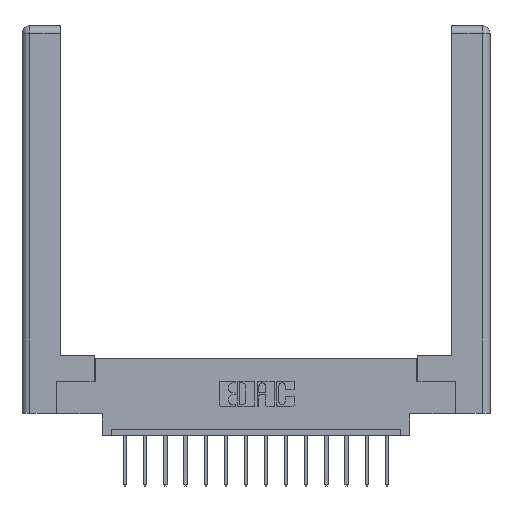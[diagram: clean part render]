
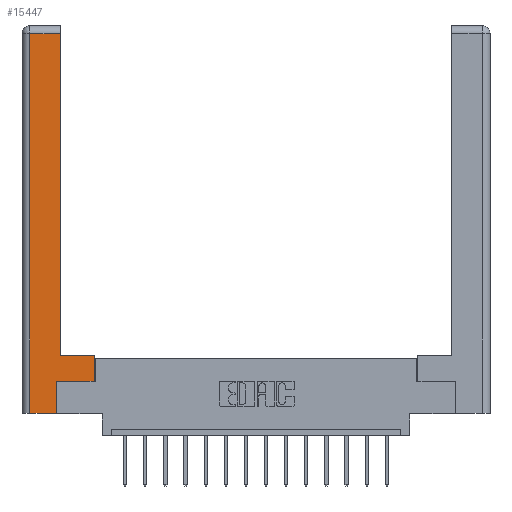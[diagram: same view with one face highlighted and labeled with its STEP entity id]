
A CAD part, top view. The second image highlights one B-rep face of the part: STEP entity #15447.
In plain terms, the highlighted planar face has unit normal (0, 0, 1).
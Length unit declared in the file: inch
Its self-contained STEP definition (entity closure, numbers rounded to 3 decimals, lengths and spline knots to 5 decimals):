
#81 = VECTOR ( 'NONE', #10114, 39.37008 ) ;
#239 = CARTESIAN_POINT ( 'NONE',  ( 0.295, 0.45, 0. ) ) ;
#407 = VECTOR ( 'NONE', #8859, 39.37008 ) ;
#455 = ORIENTED_EDGE ( 'NONE', *, *, #9936, .T. ) ;
#558 = CARTESIAN_POINT ( 'NONE',  ( 0.565, 0.45, 0. ) ) ;
#618 = EDGE_CURVE ( 'NONE', #16006, #5156, #6017, .T. ) ;
#855 = VERTEX_POINT ( 'NONE', #1150 ) ;
#1150 = CARTESIAN_POINT ( 'NONE',  ( 0.0615, 2.94, 0. ) ) ;
#1838 = LINE ( 'NONE', #3688, #6533 ) ;
#1872 = EDGE_LOOP ( 'NONE', ( #15704, #4739, #12392, #5557, #455, #7650, #2362, #10846 ) ) ;
#2362 = ORIENTED_EDGE ( 'NONE', *, *, #11841, .T. ) ;
#2445 = CARTESIAN_POINT ( 'NONE',  ( 0.265, 0.245, 0. ) ) ;
#2701 = DIRECTION ( 'NONE',  ( 0., 0., -1. ) ) ;
#2798 = CARTESIAN_POINT ( 'NONE',  ( 0.0615, 0., 0. ) ) ;
#2969 = VERTEX_POINT ( 'NONE', #16063 ) ;
#3688 = CARTESIAN_POINT ( 'NONE',  ( 0.0615, 2.94, 0. ) ) ;
#3745 = VECTOR ( 'NONE', #5831, 39.37008 ) ;
#3773 = EDGE_CURVE ( 'NONE', #5156, #10275, #3832, .T. ) ;
#3832 = LINE ( 'NONE', #8805, #407 ) ;
#4126 = VERTEX_POINT ( 'NONE', #9240 ) ;
#4253 = DIRECTION ( 'NONE',  ( 1., 0., 0. ) ) ;
#4575 = FACE_OUTER_BOUND ( 'NONE', #1872, .T. ) ;
#4739 = ORIENTED_EDGE ( 'NONE', *, *, #12572, .T. ) ;
#5156 = VERTEX_POINT ( 'NONE', #239 ) ;
#5321 = LINE ( 'NONE', #558, #6947 ) ;
#5557 = ORIENTED_EDGE ( 'NONE', *, *, #7665, .T. ) ;
#5831 = DIRECTION ( 'NONE',  ( -1., 0., 0. ) ) ;
#6017 = LINE ( 'NONE', #12247, #3745 ) ;
#6103 = DIRECTION ( 'NONE',  ( -1., 0., 0. ) ) ;
#6448 = VECTOR ( 'NONE', #11891, 39.37008 ) ;
#6533 = VECTOR ( 'NONE', #6103, 39.37008 ) ;
#6735 = PLANE ( 'NONE',  #13606 ) ;
#6946 = CARTESIAN_POINT ( 'NONE',  ( 0.565, 0.245, 0. ) ) ;
#6947 = VECTOR ( 'NONE', #7088, 39.37008 ) ;
#7088 = DIRECTION ( 'NONE',  ( 0., 1., 0. ) ) ;
#7208 = VECTOR ( 'NONE', #14643, 39.37008 ) ;
#7650 = ORIENTED_EDGE ( 'NONE', *, *, #8735, .T. ) ;
#7665 = EDGE_CURVE ( 'NONE', #9887, #2969, #7688, .T. ) ;
#7688 = LINE ( 'NONE', #12056, #9328 ) ;
#7979 = CARTESIAN_POINT ( 'NONE',  ( 0.265, 0.245, 0. ) ) ;
#8669 = LINE ( 'NONE', #6946, #6448 ) ;
#8735 = EDGE_CURVE ( 'NONE', #12671, #4126, #8669, .T. ) ;
#8805 = CARTESIAN_POINT ( 'NONE',  ( 0.295, 3., 0. ) ) ;
#8859 = DIRECTION ( 'NONE',  ( 0., 1., 0. ) ) ;
#9240 = CARTESIAN_POINT ( 'NONE',  ( 0.565, 0.245, 0. ) ) ;
#9328 = VECTOR ( 'NONE', #4253, 39.37008 ) ;
#9887 = VERTEX_POINT ( 'NONE', #2798 ) ;
#9936 = EDGE_CURVE ( 'NONE', #2969, #12671, #14561, .T. ) ;
#10114 = DIRECTION ( 'NONE',  ( 0., -1., 0. ) ) ;
#10275 = VERTEX_POINT ( 'NONE', #16827 ) ;
#10667 = DIRECTION ( 'NONE',  ( -1., 0., 0. ) ) ;
#10846 = ORIENTED_EDGE ( 'NONE', *, *, #618, .T. ) ;
#11579 = CARTESIAN_POINT ( 'NONE',  ( 0.0615, 0., 0. ) ) ;
#11841 = EDGE_CURVE ( 'NONE', #4126, #16006, #5321, .T. ) ;
#11891 = DIRECTION ( 'NONE',  ( 1., 0., 0. ) ) ;
#12056 = CARTESIAN_POINT ( 'NONE',  ( 0.265, 0., 0. ) ) ;
#12247 = CARTESIAN_POINT ( 'NONE',  ( 0.295, 0.45, 0. ) ) ;
#12392 = ORIENTED_EDGE ( 'NONE', *, *, #16426, .T. ) ;
#12468 = CARTESIAN_POINT ( 'NONE',  ( 0.565, 0.45, 0. ) ) ;
#12572 = EDGE_CURVE ( 'NONE', #10275, #855, #1838, .T. ) ;
#12671 = VERTEX_POINT ( 'NONE', #2445 ) ;
#13067 = CARTESIAN_POINT ( 'NONE',  ( 0., 0., 0. ) ) ;
#13606 = AXIS2_PLACEMENT_3D ( 'NONE', #13067, #2701, #10667 ) ;
#13729 = LINE ( 'NONE', #11579, #81 ) ;
#14561 = LINE ( 'NONE', #7979, #7208 ) ;
#14643 = DIRECTION ( 'NONE',  ( 0., 1., 0. ) ) ;
#15447 = ADVANCED_FACE ( 'NONE', ( #4575 ), #6735, .F. ) ;
#15704 = ORIENTED_EDGE ( 'NONE', *, *, #3773, .T. ) ;
#16006 = VERTEX_POINT ( 'NONE', #12468 ) ;
#16063 = CARTESIAN_POINT ( 'NONE',  ( 0.265, 0., 0. ) ) ;
#16426 = EDGE_CURVE ( 'NONE', #855, #9887, #13729, .T. ) ;
#16827 = CARTESIAN_POINT ( 'NONE',  ( 0.295, 2.94, 0. ) ) ;
